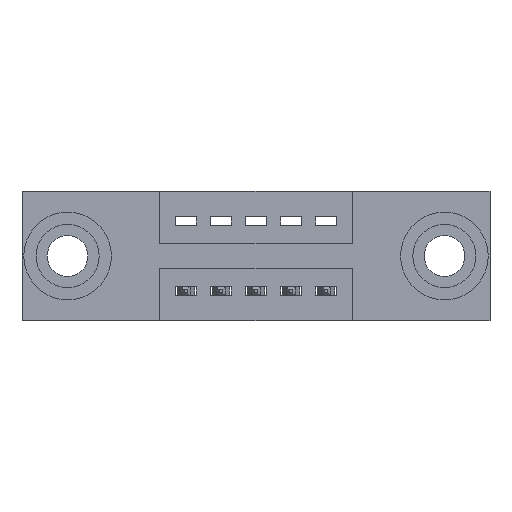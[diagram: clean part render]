
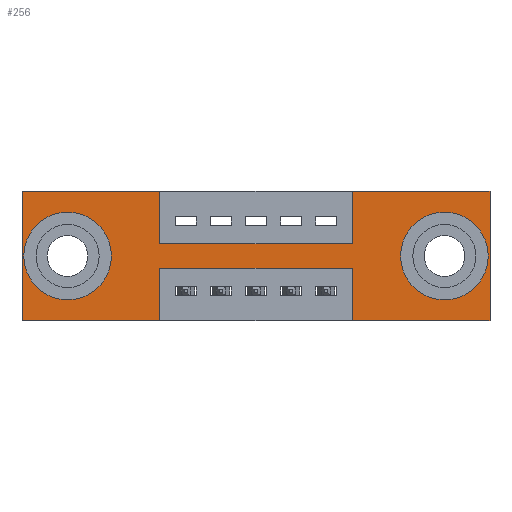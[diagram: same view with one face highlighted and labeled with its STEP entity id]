
A CAD part, front view. The second image highlights one B-rep face of the part: STEP entity #256.
In plain terms, the highlighted planar face has unit normal (0, -1, 0).
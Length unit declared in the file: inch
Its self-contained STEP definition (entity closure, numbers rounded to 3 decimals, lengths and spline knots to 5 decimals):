
#21 = AXIS2_PLACEMENT_3D ( 'NONE', #1298, #3480, #7883 ) ;
#22 = LINE ( 'NONE', #4248, #8867 ) ;
#86 = CARTESIAN_POINT ( 'NONE',  ( 0., 0., -0.37 ) ) ;
#221 = DIRECTION ( 'NONE',  ( 1., 0., 0. ) ) ;
#249 = VERTEX_POINT ( 'NONE', #3853 ) ;
#256 = ADVANCED_FACE ( 'NONE', ( #610, #3539, #4241 ), #1770, .T. ) ;
#276 = CIRCLE ( 'NONE', #21, 0.078 ) ;
#334 = LINE ( 'NONE', #892, #2037 ) ;
#420 = CARTESIAN_POINT ( 'NONE',  ( 0.9425, 0., -0.22 ) ) ;
#610 = FACE_BOUND ( 'NONE', #2366, .T. ) ;
#620 = LINE ( 'NONE', #7310, #8113 ) ;
#637 = VERTEX_POINT ( 'NONE', #9308 ) ;
#752 = DIRECTION ( 'NONE',  ( 0., 0., -1. ) ) ;
#854 = EDGE_CURVE ( 'NONE', #5467, #7852, #6982, .T. ) ;
#892 = CARTESIAN_POINT ( 'NONE',  ( 0., 0., 0. ) ) ;
#914 = EDGE_LOOP ( 'NONE', ( #5889, #8724 ) ) ;
#919 = LINE ( 'NONE', #1568, #4550 ) ;
#1011 = VERTEX_POINT ( 'NONE', #1970 ) ;
#1093 = CARTESIAN_POINT ( 'NONE',  ( 0.9425, 0., 0. ) ) ;
#1094 = CARTESIAN_POINT ( 'NONE',  ( 0.13, 0., -0.185 ) ) ;
#1109 = EDGE_CURVE ( 'NONE', #2982, #3484, #5342, .T. ) ;
#1253 = ORIENTED_EDGE ( 'NONE', *, *, #3303, .F. ) ;
#1298 = CARTESIAN_POINT ( 'NONE',  ( 0.13, 0., -0.185 ) ) ;
#1313 = ORIENTED_EDGE ( 'NONE', *, *, #2325, .F. ) ;
#1359 = DIRECTION ( 'NONE',  ( 0., 0., -1. ) ) ;
#1373 = EDGE_CURVE ( 'NONE', #7846, #2155, #919, .T. ) ;
#1528 = VERTEX_POINT ( 'NONE', #4663 ) ;
#1568 = CARTESIAN_POINT ( 'NONE',  ( 0.3925, 0., -0.22 ) ) ;
#1764 = LINE ( 'NONE', #4514, #2004 ) ;
#1770 = PLANE ( 'NONE',  #4981 ) ;
#1788 = AXIS2_PLACEMENT_3D ( 'NONE', #2059, #4295, #4322 ) ;
#1860 = EDGE_CURVE ( 'NONE', #2155, #5507, #22, .T. ) ;
#1941 = ORIENTED_EDGE ( 'NONE', *, *, #6988, .T. ) ;
#1970 = CARTESIAN_POINT ( 'NONE',  ( 1.335, 0., -0.37 ) ) ;
#2004 = VECTOR ( 'NONE', #4478, 39.37008 ) ;
#2037 = VECTOR ( 'NONE', #7381, 39.37008 ) ;
#2059 = CARTESIAN_POINT ( 'NONE',  ( 1.205, 0., -0.185 ) ) ;
#2097 = ORIENTED_EDGE ( 'NONE', *, *, #5769, .F. ) ;
#2123 = DIRECTION ( 'NONE',  ( -1., 0., 0. ) ) ;
#2155 = VERTEX_POINT ( 'NONE', #2203 ) ;
#2203 = CARTESIAN_POINT ( 'NONE',  ( 0.3925, 0., -0.22 ) ) ;
#2223 = DIRECTION ( 'NONE',  ( 1., 0., 0. ) ) ;
#2325 = EDGE_CURVE ( 'NONE', #7852, #7879, #3393, .T. ) ;
#2337 = CARTESIAN_POINT ( 'NONE',  ( 0., 0., -0.37 ) ) ;
#2366 = EDGE_LOOP ( 'NONE', ( #5372, #1941 ) ) ;
#2673 = VECTOR ( 'NONE', #2123, 39.37008 ) ;
#2718 = VECTOR ( 'NONE', #221, 39.37008 ) ;
#2982 = VERTEX_POINT ( 'NONE', #6267 ) ;
#3070 = VECTOR ( 'NONE', #3169, 39.37008 ) ;
#3169 = DIRECTION ( 'NONE',  ( 1., 0., 0. ) ) ;
#3171 = LINE ( 'NONE', #6833, #3070 ) ;
#3303 = EDGE_CURVE ( 'NONE', #1528, #637, #1764, .T. ) ;
#3370 = CARTESIAN_POINT ( 'NONE',  ( 0.3925, 0., -0.37 ) ) ;
#3380 = EDGE_CURVE ( 'NONE', #8420, #249, #4392, .T. ) ;
#3393 = LINE ( 'NONE', #4532, #2718 ) ;
#3459 = DIRECTION ( 'NONE',  ( -1., 0., 0. ) ) ;
#3480 = DIRECTION ( 'NONE',  ( 0., 1., 0. ) ) ;
#3484 = VERTEX_POINT ( 'NONE', #7577 ) ;
#3537 = CARTESIAN_POINT ( 'NONE',  ( 1.205, 0., -0.185 ) ) ;
#3539 = FACE_BOUND ( 'NONE', #914, .T. ) ;
#3646 = ORIENTED_EDGE ( 'NONE', *, *, #6390, .F. ) ;
#3790 = LINE ( 'NONE', #86, #2673 ) ;
#3791 = VERTEX_POINT ( 'NONE', #7625 ) ;
#3825 = DIRECTION ( 'NONE',  ( 0., 0., -1. ) ) ;
#3853 = CARTESIAN_POINT ( 'NONE',  ( 0.13, 0., -0.263 ) ) ;
#4166 = ORIENTED_EDGE ( 'NONE', *, *, #8071, .F. ) ;
#4241 = FACE_OUTER_BOUND ( 'NONE', #4474, .T. ) ;
#4248 = CARTESIAN_POINT ( 'NONE',  ( 0.3925, 0., -0.37 ) ) ;
#4295 = DIRECTION ( 'NONE',  ( 0., 1., 0. ) ) ;
#4322 = DIRECTION ( 'NONE',  ( 0., 0., -1. ) ) ;
#4377 = VECTOR ( 'NONE', #3459, 39.37008 ) ;
#4392 = CIRCLE ( 'NONE', #7518, 0.078 ) ;
#4474 = EDGE_LOOP ( 'NONE', ( #8828, #6908, #9259, #2097, #7212, #1313, #5404, #4166, #1253, #3646, #6200, #6611 ) ) ;
#4478 = DIRECTION ( 'NONE',  ( 0., 0., -1. ) ) ;
#4514 = CARTESIAN_POINT ( 'NONE',  ( 0.3925, 0., 0. ) ) ;
#4532 = CARTESIAN_POINT ( 'NONE',  ( 0., 0., 0. ) ) ;
#4550 = VECTOR ( 'NONE', #6819, 39.37008 ) ;
#4663 = CARTESIAN_POINT ( 'NONE',  ( 0.3925, 0., 0. ) ) ;
#4981 = AXIS2_PLACEMENT_3D ( 'NONE', #7604, #6887, #3825 ) ;
#5087 = CARTESIAN_POINT ( 'NONE',  ( 1.335, 0., 0. ) ) ;
#5228 = CARTESIAN_POINT ( 'NONE',  ( 0.9425, 0., -0.37 ) ) ;
#5262 = DIRECTION ( 'NONE',  ( 0., 0., 1. ) ) ;
#5342 = CIRCLE ( 'NONE', #1788, 0.078 ) ;
#5362 = CIRCLE ( 'NONE', #6607, 0.078 ) ;
#5372 = ORIENTED_EDGE ( 'NONE', *, *, #1109, .T. ) ;
#5381 = VERTEX_POINT ( 'NONE', #2337 ) ;
#5404 = ORIENTED_EDGE ( 'NONE', *, *, #854, .F. ) ;
#5467 = VERTEX_POINT ( 'NONE', #7445 ) ;
#5501 = VECTOR ( 'NONE', #752, 39.37008 ) ;
#5507 = VERTEX_POINT ( 'NONE', #3370 ) ;
#5714 = DIRECTION ( 'NONE',  ( 0., 1., 0. ) ) ;
#5738 = EDGE_CURVE ( 'NONE', #5507, #5381, #6337, .T. ) ;
#5769 = EDGE_CURVE ( 'NONE', #1011, #7156, #3790, .T. ) ;
#5796 = LINE ( 'NONE', #5228, #5917 ) ;
#5889 = ORIENTED_EDGE ( 'NONE', *, *, #3380, .T. ) ;
#5902 = CARTESIAN_POINT ( 'NONE',  ( 1.335, 0., 0. ) ) ;
#5917 = VECTOR ( 'NONE', #5262, 39.37008 ) ;
#6200 = ORIENTED_EDGE ( 'NONE', *, *, #9269, .F. ) ;
#6267 = CARTESIAN_POINT ( 'NONE',  ( 1.205, 0., -0.107 ) ) ;
#6337 = LINE ( 'NONE', #7839, #4377 ) ;
#6356 = EDGE_CURVE ( 'NONE', #249, #8420, #276, .T. ) ;
#6390 = EDGE_CURVE ( 'NONE', #3791, #1528, #620, .T. ) ;
#6408 = EDGE_CURVE ( 'NONE', #7879, #1011, #7431, .T. ) ;
#6607 = AXIS2_PLACEMENT_3D ( 'NONE', #3537, #5714, #1359 ) ;
#6611 = ORIENTED_EDGE ( 'NONE', *, *, #5738, .F. ) ;
#6744 = VECTOR ( 'NONE', #9112, 39.37008 ) ;
#6819 = DIRECTION ( 'NONE',  ( -1., 0., 0. ) ) ;
#6833 = CARTESIAN_POINT ( 'NONE',  ( 0.3925, 0., -0.15 ) ) ;
#6887 = DIRECTION ( 'NONE',  ( 0., -1., 0. ) ) ;
#6908 = ORIENTED_EDGE ( 'NONE', *, *, #1373, .F. ) ;
#6982 = LINE ( 'NONE', #1093, #6744 ) ;
#6988 = EDGE_CURVE ( 'NONE', #3484, #2982, #5362, .T. ) ;
#7156 = VERTEX_POINT ( 'NONE', #8448 ) ;
#7212 = ORIENTED_EDGE ( 'NONE', *, *, #6408, .F. ) ;
#7310 = CARTESIAN_POINT ( 'NONE',  ( 0., 0., 0. ) ) ;
#7381 = DIRECTION ( 'NONE',  ( 0., 0., 1. ) ) ;
#7431 = LINE ( 'NONE', #5087, #5501 ) ;
#7445 = CARTESIAN_POINT ( 'NONE',  ( 0.9425, 0., -0.15 ) ) ;
#7518 = AXIS2_PLACEMENT_3D ( 'NONE', #1094, #8378, #8339 ) ;
#7577 = CARTESIAN_POINT ( 'NONE',  ( 1.205, 0., -0.263 ) ) ;
#7604 = CARTESIAN_POINT ( 'NONE',  ( 0., 0., -0.37 ) ) ;
#7625 = CARTESIAN_POINT ( 'NONE',  ( 0., 0., 0. ) ) ;
#7628 = CARTESIAN_POINT ( 'NONE',  ( 0.9425, 0., 0. ) ) ;
#7839 = CARTESIAN_POINT ( 'NONE',  ( 0., 0., -0.37 ) ) ;
#7846 = VERTEX_POINT ( 'NONE', #420 ) ;
#7852 = VERTEX_POINT ( 'NONE', #7628 ) ;
#7879 = VERTEX_POINT ( 'NONE', #5902 ) ;
#7883 = DIRECTION ( 'NONE',  ( 0., 0., 1. ) ) ;
#8071 = EDGE_CURVE ( 'NONE', #637, #5467, #3171, .T. ) ;
#8113 = VECTOR ( 'NONE', #2223, 39.37008 ) ;
#8143 = CARTESIAN_POINT ( 'NONE',  ( 0.13, 0., -0.107 ) ) ;
#8339 = DIRECTION ( 'NONE',  ( 0., 0., 1. ) ) ;
#8378 = DIRECTION ( 'NONE',  ( 0., 1., 0. ) ) ;
#8420 = VERTEX_POINT ( 'NONE', #8143 ) ;
#8448 = CARTESIAN_POINT ( 'NONE',  ( 0.9425, 0., -0.37 ) ) ;
#8585 = DIRECTION ( 'NONE',  ( 0., 0., -1. ) ) ;
#8701 = EDGE_CURVE ( 'NONE', #7156, #7846, #5796, .T. ) ;
#8724 = ORIENTED_EDGE ( 'NONE', *, *, #6356, .T. ) ;
#8828 = ORIENTED_EDGE ( 'NONE', *, *, #1860, .F. ) ;
#8867 = VECTOR ( 'NONE', #8585, 39.37008 ) ;
#9112 = DIRECTION ( 'NONE',  ( 0., 0., 1. ) ) ;
#9259 = ORIENTED_EDGE ( 'NONE', *, *, #8701, .F. ) ;
#9269 = EDGE_CURVE ( 'NONE', #5381, #3791, #334, .T. ) ;
#9308 = CARTESIAN_POINT ( 'NONE',  ( 0.3925, 0., -0.15 ) ) ;
